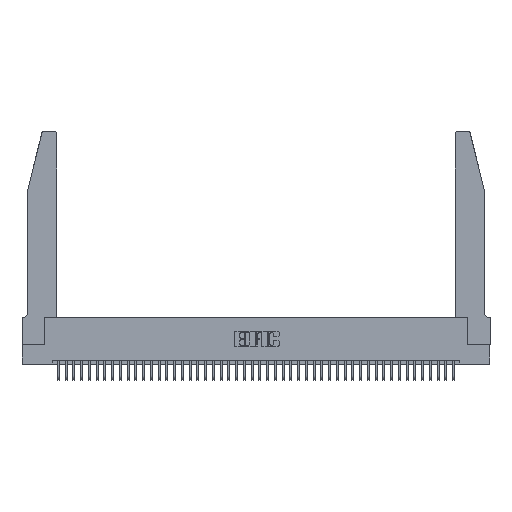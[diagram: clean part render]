
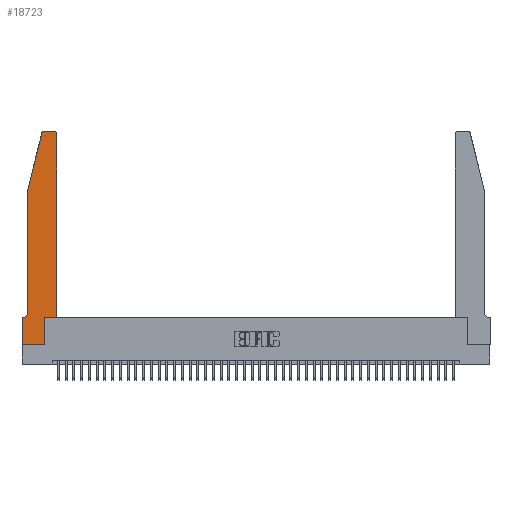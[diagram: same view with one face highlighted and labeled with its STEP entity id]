
A CAD part, top view. The second image highlights one B-rep face of the part: STEP entity #18723.
In plain terms, the highlighted planar face has unit normal (0, 0, 1).
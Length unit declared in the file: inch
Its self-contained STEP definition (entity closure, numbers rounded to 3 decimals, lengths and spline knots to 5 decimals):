
#272 = CARTESIAN_POINT ( 'NONE',  ( 0.0055, 0.42, 0.37 ) ) ;
#1332 = CARTESIAN_POINT ( 'NONE',  ( 0.2865, 0., 0.37 ) ) ;
#2014 = CARTESIAN_POINT ( 'NONE',  ( 0.4205, 2.72, 0.37 ) ) ;
#2581 = VECTOR ( 'NONE', #24039, 39.37008 ) ;
#2590 = ORIENTED_EDGE ( 'NONE', *, *, #32245, .T. ) ;
#2623 = CARTESIAN_POINT ( 'NONE',  ( 0.4505, 2.72, 0.37 ) ) ;
#2737 = EDGE_CURVE ( 'NONE', #13772, #40520, #41374, .T. ) ;
#3442 = DIRECTION ( 'NONE',  ( -1., 0., 0. ) ) ;
#3957 = DIRECTION ( 'NONE',  ( -1., 0., 0. ) ) ;
#5707 = DIRECTION ( 'NONE',  ( 1., 0., 0. ) ) ;
#6565 = CARTESIAN_POINT ( 'NONE',  ( 0.0755, 2., 0.37 ) ) ;
#6801 = CARTESIAN_POINT ( 'NONE',  ( 0.2865, 0.35, 0.37 ) ) ;
#7034 = DIRECTION ( 'NONE',  ( -1., 0., 0. ) ) ;
#7245 = AXIS2_PLACEMENT_3D ( 'NONE', #14047, #10606, #35295 ) ;
#7475 = CARTESIAN_POINT ( 'NONE',  ( 0.284, 2.72, 0.37 ) ) ;
#7619 = CARTESIAN_POINT ( 'NONE',  ( 0., 0., 0.37 ) ) ;
#8843 = ORIENTED_EDGE ( 'NONE', *, *, #32845, .T. ) ;
#9091 = AXIS2_PLACEMENT_3D ( 'NONE', #7475, #32255, #11060 ) ;
#9131 = EDGE_CURVE ( 'NONE', #39185, #35343, #43615, .T. ) ;
#10163 = CARTESIAN_POINT ( 'NONE',  ( 0.25487, 2.72718, 0.37 ) ) ;
#10606 = DIRECTION ( 'NONE',  ( 0., 0., 1. ) ) ;
#11024 = ORIENTED_EDGE ( 'NONE', *, *, #20689, .T. ) ;
#11060 = DIRECTION ( 'NONE',  ( 1., 0., 0. ) ) ;
#11440 = CARTESIAN_POINT ( 'NONE',  ( 0.2865, 0.35, 0.37 ) ) ;
#11591 = ORIENTED_EDGE ( 'NONE', *, *, #30140, .T. ) ;
#12610 = CARTESIAN_POINT ( 'NONE',  ( 0.4205, 2.75, 0.37 ) ) ;
#13772 = VERTEX_POINT ( 'NONE', #16218 ) ;
#13904 = LINE ( 'NONE', #23793, #31568 ) ;
#14047 = CARTESIAN_POINT ( 'NONE',  ( 0., 0.35, 0.37 ) ) ;
#14478 = EDGE_CURVE ( 'NONE', #30546, #40334, #41067, .T. ) ;
#15577 = AXIS2_PLACEMENT_3D ( 'NONE', #2014, #26967, #5707 ) ;
#16218 = CARTESIAN_POINT ( 'NONE',  ( 0.0755, 2., 0.37 ) ) ;
#17013 = VECTOR ( 'NONE', #42953, 39.37008 ) ;
#17190 = CARTESIAN_POINT ( 'NONE',  ( 0.4505, 0.35, 0.37 ) ) ;
#18723 = ADVANCED_FACE ( 'NONE', ( #41082 ), #31783, .T. ) ;
#19231 = VECTOR ( 'NONE', #7034, 39.37008 ) ;
#19332 = ORIENTED_EDGE ( 'NONE', *, *, #20695, .T. ) ;
#20023 = VERTEX_POINT ( 'NONE', #35812 ) ;
#20689 = EDGE_CURVE ( 'NONE', #41916, #13772, #34841, .T. ) ;
#20695 = EDGE_CURVE ( 'NONE', #20023, #41916, #25494, .T. ) ;
#20867 = DIRECTION ( 'NONE',  ( 0., -1., 0. ) ) ;
#21143 = LINE ( 'NONE', #35382, #38756 ) ;
#21572 = VERTEX_POINT ( 'NONE', #45373 ) ;
#21624 = ORIENTED_EDGE ( 'NONE', *, *, #14478, .T. ) ;
#22644 = DIRECTION ( 'NONE',  ( 0., 1., 0. ) ) ;
#22706 = CARTESIAN_POINT ( 'NONE',  ( 0., 0.35, 0.37 ) ) ;
#23259 = DIRECTION ( 'NONE',  ( 1., 0., 0. ) ) ;
#23793 = CARTESIAN_POINT ( 'NONE',  ( 0., 0., 0.37 ) ) ;
#23822 = VECTOR ( 'NONE', #23259, 39.37008 ) ;
#24039 = DIRECTION ( 'NONE',  ( 0., 1., 0. ) ) ;
#24343 = ORIENTED_EDGE ( 'NONE', *, *, #43697, .T. ) ;
#24650 = VERTEX_POINT ( 'NONE', #25541 ) ;
#24718 = CARTESIAN_POINT ( 'NONE',  ( 0.0755, 0.35, 0.37 ) ) ;
#25272 = DIRECTION ( 'NONE',  ( 0., 0., -1. ) ) ;
#25494 = CIRCLE ( 'NONE', #9091, 0.03 ) ;
#25541 = CARTESIAN_POINT ( 'NONE',  ( 0.0055, 0.35, 0.37 ) ) ;
#26423 = LINE ( 'NONE', #7619, #17013 ) ;
#26967 = DIRECTION ( 'NONE',  ( 0., 0., 1. ) ) ;
#27171 = LINE ( 'NONE', #40182, #35428 ) ;
#27299 = CIRCLE ( 'NONE', #31868, 0.07 ) ;
#28398 = EDGE_CURVE ( 'NONE', #24650, #44134, #40176, .T. ) ;
#30140 = EDGE_CURVE ( 'NONE', #40520, #24650, #27299, .T. ) ;
#30361 = CARTESIAN_POINT ( 'NONE',  ( 0.4505, 0.35, 0.37 ) ) ;
#30546 = VERTEX_POINT ( 'NONE', #2623 ) ;
#30896 = DIRECTION ( 'NONE',  ( 0., -1., 0. ) ) ;
#31306 = CARTESIAN_POINT ( 'NONE',  ( 0.0755, 0.42, 0.37 ) ) ;
#31568 = VECTOR ( 'NONE', #30896, 39.37008 ) ;
#31740 = EDGE_LOOP ( 'NONE', ( #34769, #19332, #11024, #38666, #11591, #41938, #24343, #35916, #8843, #36991, #2590, #21624 ) ) ;
#31783 = PLANE ( 'NONE',  #7245 ) ;
#31868 = AXIS2_PLACEMENT_3D ( 'NONE', #272, #25272, #3957 ) ;
#32066 = VECTOR ( 'NONE', #20867, 39.37008 ) ;
#32245 = EDGE_CURVE ( 'NONE', #35343, #30546, #27171, .T. ) ;
#32255 = DIRECTION ( 'NONE',  ( 0., 0., 1. ) ) ;
#32845 = EDGE_CURVE ( 'NONE', #39585, #39185, #40309, .T. ) ;
#34290 = EDGE_CURVE ( 'NONE', #21572, #39585, #26423, .T. ) ;
#34769 = ORIENTED_EDGE ( 'NONE', *, *, #37790, .T. ) ;
#34841 = LINE ( 'NONE', #35614, #43054 ) ;
#35295 = DIRECTION ( 'NONE',  ( 1., 0., 0. ) ) ;
#35343 = VERTEX_POINT ( 'NONE', #17190 ) ;
#35382 = CARTESIAN_POINT ( 'NONE',  ( 0.2605, 2.75, 0.37 ) ) ;
#35428 = VECTOR ( 'NONE', #22644, 39.37008 ) ;
#35614 = CARTESIAN_POINT ( 'NONE',  ( 0.0755, 2., 0.37 ) ) ;
#35812 = CARTESIAN_POINT ( 'NONE',  ( 0.284, 2.75, 0.37 ) ) ;
#35916 = ORIENTED_EDGE ( 'NONE', *, *, #34290, .T. ) ;
#36991 = ORIENTED_EDGE ( 'NONE', *, *, #9131, .T. ) ;
#37790 = EDGE_CURVE ( 'NONE', #40334, #20023, #21143, .T. ) ;
#38666 = ORIENTED_EDGE ( 'NONE', *, *, #2737, .T. ) ;
#38756 = VECTOR ( 'NONE', #3442, 39.37008 ) ;
#39154 = DIRECTION ( 'NONE',  ( -0.239, -0.971, 0. ) ) ;
#39185 = VERTEX_POINT ( 'NONE', #6801 ) ;
#39585 = VERTEX_POINT ( 'NONE', #1332 ) ;
#40176 = LINE ( 'NONE', #24718, #19231 ) ;
#40182 = CARTESIAN_POINT ( 'NONE',  ( 0.4505, 0.35, 0.37 ) ) ;
#40309 = LINE ( 'NONE', #11440, #2581 ) ;
#40334 = VERTEX_POINT ( 'NONE', #12610 ) ;
#40520 = VERTEX_POINT ( 'NONE', #31306 ) ;
#41067 = CIRCLE ( 'NONE', #15577, 0.03 ) ;
#41082 = FACE_OUTER_BOUND ( 'NONE', #31740, .T. ) ;
#41374 = LINE ( 'NONE', #6565, #32066 ) ;
#41916 = VERTEX_POINT ( 'NONE', #10163 ) ;
#41938 = ORIENTED_EDGE ( 'NONE', *, *, #28398, .T. ) ;
#42953 = DIRECTION ( 'NONE',  ( 1., 0., 0. ) ) ;
#43054 = VECTOR ( 'NONE', #39154, 39.37008 ) ;
#43615 = LINE ( 'NONE', #30361, #23822 ) ;
#43697 = EDGE_CURVE ( 'NONE', #44134, #21572, #13904, .T. ) ;
#44134 = VERTEX_POINT ( 'NONE', #22706 ) ;
#45373 = CARTESIAN_POINT ( 'NONE',  ( 0., 0., 0.37 ) ) ;
